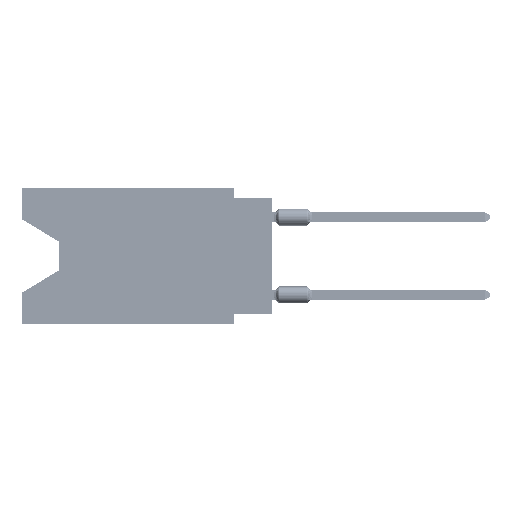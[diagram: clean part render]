
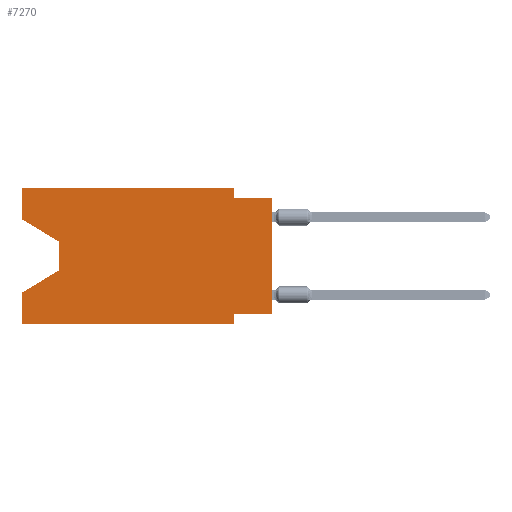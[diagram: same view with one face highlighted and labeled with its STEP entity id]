
A CAD part, left-side view. The second image highlights one B-rep face of the part: STEP entity #7270.
In plain terms, the highlighted planar face has unit normal (-1, 0, 0).
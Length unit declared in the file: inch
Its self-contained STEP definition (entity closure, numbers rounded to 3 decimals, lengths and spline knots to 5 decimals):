
#1113 = EDGE_CURVE ( 'NONE', #94918, #62669, #101940, .T. ) ;
#1185 = CARTESIAN_POINT ( 'NONE',  ( 0., 0.55, -0.138 ) ) ;
#1363 = VECTOR ( 'NONE', #18873, 39.37008 ) ;
#1933 = EDGE_CURVE ( 'NONE', #36659, #50266, #97442, .T. ) ;
#2240 = CARTESIAN_POINT ( 'NONE',  ( 0., 0.645, 0. ) ) ;
#3291 = CARTESIAN_POINT ( 'NONE',  ( 0., 0., -0.025 ) ) ;
#3871 = ORIENTED_EDGE ( 'NONE', *, *, #1113, .T. ) ;
#4347 = LINE ( 'NONE', #104744, #12236 ) ;
#5388 = CARTESIAN_POINT ( 'NONE',  ( 0., 0., -0.325 ) ) ;
#5986 = EDGE_CURVE ( 'NONE', #17134, #65469, #4347, .T. ) ;
#7025 = DIRECTION ( 'NONE',  ( 1., 0., 0. ) ) ;
#7270 = ADVANCED_FACE ( 'NONE', ( #56664 ), #31046, .F. ) ;
#8942 = EDGE_CURVE ( 'NONE', #51402, #98241, #18603, .T. ) ;
#9988 = CARTESIAN_POINT ( 'NONE',  ( 0., 0.1, -0.35 ) ) ;
#11532 = VECTOR ( 'NONE', #61294, 39.37008 ) ;
#12025 = EDGE_CURVE ( 'NONE', #57147, #65469, #102409, .T. ) ;
#12236 = VECTOR ( 'NONE', #78582, 39.37008 ) ;
#17134 = VERTEX_POINT ( 'NONE', #5388 ) ;
#17819 = VECTOR ( 'NONE', #35483, 39.37008 ) ;
#17877 = DIRECTION ( 'NONE',  ( 0., -1., 0. ) ) ;
#18603 = LINE ( 'NONE', #2240, #17819 ) ;
#18873 = DIRECTION ( 'NONE',  ( 0., 0., -1. ) ) ;
#19972 = DIRECTION ( 'NONE',  ( 0., -1., 0. ) ) ;
#20457 = EDGE_CURVE ( 'NONE', #85332, #51402, #76614, .T. ) ;
#20727 = CARTESIAN_POINT ( 'NONE',  ( 0., 0., -0.325 ) ) ;
#21898 = CARTESIAN_POINT ( 'NONE',  ( 0., 0.645, -0.35 ) ) ;
#22580 = EDGE_CURVE ( 'NONE', #85332, #36659, #97534, .T. ) ;
#26365 = ORIENTED_EDGE ( 'NONE', *, *, #1933, .T. ) ;
#26996 = ORIENTED_EDGE ( 'NONE', *, *, #20457, .F. ) ;
#28731 = VERTEX_POINT ( 'NONE', #98569 ) ;
#29243 = DIRECTION ( 'NONE',  ( 0., 0., -1. ) ) ;
#31046 = PLANE ( 'NONE',  #71786 ) ;
#33132 = ORIENTED_EDGE ( 'NONE', *, *, #8942, .F. ) ;
#33172 = EDGE_CURVE ( 'NONE', #28731, #62669, #50889, .T. ) ;
#33614 = CARTESIAN_POINT ( 'NONE',  ( 0., 0.645, 0. ) ) ;
#34472 = CARTESIAN_POINT ( 'NONE',  ( 0., 0.55, -0.212 ) ) ;
#34523 = DIRECTION ( 'NONE',  ( 0., 0., -1. ) ) ;
#35483 = DIRECTION ( 'NONE',  ( 0., -1., 0. ) ) ;
#35880 = CARTESIAN_POINT ( 'NONE',  ( 0., 0.645, -0.35 ) ) ;
#36659 = VERTEX_POINT ( 'NONE', #1185 ) ;
#37380 = LINE ( 'NONE', #70705, #1363 ) ;
#37514 = VECTOR ( 'NONE', #19972, 39.37008 ) ;
#38185 = LINE ( 'NONE', #71493, #79766 ) ;
#43202 = ORIENTED_EDGE ( 'NONE', *, *, #22580, .T. ) ;
#43415 = CARTESIAN_POINT ( 'NONE',  ( 0., 0.1, -0.025 ) ) ;
#46656 = ORIENTED_EDGE ( 'NONE', *, *, #107612, .F. ) ;
#48929 = CARTESIAN_POINT ( 'NONE',  ( 0., 0.645, -0.08025 ) ) ;
#50266 = VERTEX_POINT ( 'NONE', #79429 ) ;
#50889 = LINE ( 'NONE', #9988, #79743 ) ;
#51402 = VERTEX_POINT ( 'NONE', #33614 ) ;
#52734 = ORIENTED_EDGE ( 'NONE', *, *, #33172, .F. ) ;
#52797 = VECTOR ( 'NONE', #17877, 39.37008 ) ;
#54747 = VECTOR ( 'NONE', #29243, 39.37008 ) ;
#56664 = FACE_OUTER_BOUND ( 'NONE', #97171, .T. ) ;
#57147 = VERTEX_POINT ( 'NONE', #43415 ) ;
#57193 = CARTESIAN_POINT ( 'NONE',  ( 0., 0.645, 0. ) ) ;
#57984 = ORIENTED_EDGE ( 'NONE', *, *, #12025, .F. ) ;
#60213 = CARTESIAN_POINT ( 'NONE',  ( 0., 0.645, 0. ) ) ;
#61294 = DIRECTION ( 'NONE',  ( 0., 0., 1. ) ) ;
#62669 = VERTEX_POINT ( 'NONE', #100768 ) ;
#62721 = DIRECTION ( 'NONE',  ( 0., 1., 0. ) ) ;
#63686 = EDGE_CURVE ( 'NONE', #94918, #85273, #38185, .T. ) ;
#65469 = VERTEX_POINT ( 'NONE', #3291 ) ;
#67767 = DIRECTION ( 'NONE',  ( 0., 0.855, -0.519 ) ) ;
#70705 = CARTESIAN_POINT ( 'NONE',  ( 0., 0.1, 0. ) ) ;
#71333 = VECTOR ( 'NONE', #89333, 39.37008 ) ;
#71493 = CARTESIAN_POINT ( 'NONE',  ( 0., 0.645, 0. ) ) ;
#71786 = AXIS2_PLACEMENT_3D ( 'NONE', #57193, #7025, #90530 ) ;
#72497 = EDGE_CURVE ( 'NONE', #17134, #28731, #96585, .T. ) ;
#74055 = CARTESIAN_POINT ( 'NONE',  ( 0., 0.645, -0.26975 ) ) ;
#74260 = VECTOR ( 'NONE', #67767, 39.37008 ) ;
#76614 = LINE ( 'NONE', #60213, #11532 ) ;
#77856 = CARTESIAN_POINT ( 'NONE',  ( 0., 0., -0.025 ) ) ;
#78582 = DIRECTION ( 'NONE',  ( 0., 0., 1. ) ) ;
#79429 = CARTESIAN_POINT ( 'NONE',  ( 0., 0.55, -0.212 ) ) ;
#79743 = VECTOR ( 'NONE', #34523, 39.37008 ) ;
#79766 = VECTOR ( 'NONE', #104801, 39.37008 ) ;
#80807 = VECTOR ( 'NONE', #62721, 39.37008 ) ;
#82547 = LINE ( 'NONE', #34472, #74260 ) ;
#84934 = ORIENTED_EDGE ( 'NONE', *, *, #72497, .F. ) ;
#85273 = VERTEX_POINT ( 'NONE', #74055 ) ;
#85332 = VERTEX_POINT ( 'NONE', #48929 ) ;
#89333 = DIRECTION ( 'NONE',  ( 0., -0.855, -0.519 ) ) ;
#90530 = DIRECTION ( 'NONE',  ( 0., 0., -1. ) ) ;
#94918 = VERTEX_POINT ( 'NONE', #21898 ) ;
#96217 = ORIENTED_EDGE ( 'NONE', *, *, #63686, .F. ) ;
#96470 = CARTESIAN_POINT ( 'NONE',  ( 0., 0.645, -0.08025 ) ) ;
#96585 = LINE ( 'NONE', #20727, #80807 ) ;
#97171 = EDGE_LOOP ( 'NONE', ( #43202, #26365, #97674, #96217, #3871, #52734, #84934, #98780, #57984, #46656, #33132, #26996 ) ) ;
#97343 = CARTESIAN_POINT ( 'NONE',  ( 0., 0.1, 0. ) ) ;
#97442 = LINE ( 'NONE', #106140, #54747 ) ;
#97534 = LINE ( 'NONE', #96470, #71333 ) ;
#97674 = ORIENTED_EDGE ( 'NONE', *, *, #102075, .T. ) ;
#98241 = VERTEX_POINT ( 'NONE', #97343 ) ;
#98569 = CARTESIAN_POINT ( 'NONE',  ( 0., 0.1, -0.325 ) ) ;
#98780 = ORIENTED_EDGE ( 'NONE', *, *, #5986, .T. ) ;
#100768 = CARTESIAN_POINT ( 'NONE',  ( 0., 0.1, -0.35 ) ) ;
#101940 = LINE ( 'NONE', #35880, #52797 ) ;
#102075 = EDGE_CURVE ( 'NONE', #50266, #85273, #82547, .T. ) ;
#102409 = LINE ( 'NONE', #77856, #37514 ) ;
#104744 = CARTESIAN_POINT ( 'NONE',  ( 0., 0., 0. ) ) ;
#104801 = DIRECTION ( 'NONE',  ( 0., 0., 1. ) ) ;
#106140 = CARTESIAN_POINT ( 'NONE',  ( 0., 0.55, -0.138 ) ) ;
#107612 = EDGE_CURVE ( 'NONE', #98241, #57147, #37380, .T. ) ;
